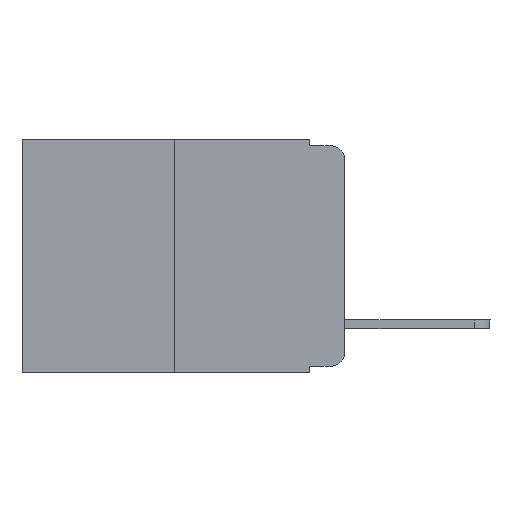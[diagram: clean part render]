
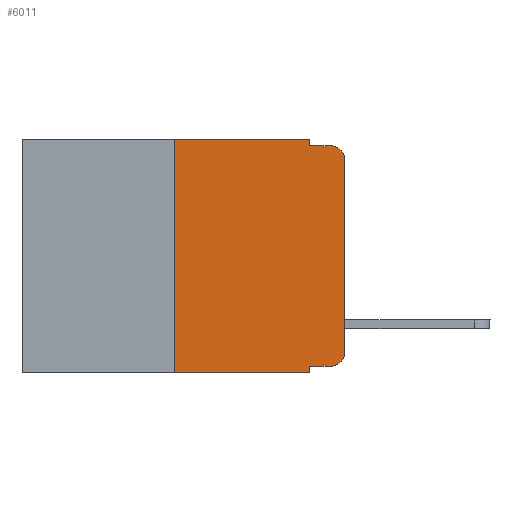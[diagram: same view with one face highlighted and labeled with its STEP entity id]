
A CAD part, left-side view. The second image highlights one B-rep face of the part: STEP entity #6011.
In plain terms, the highlighted planar face has unit normal (-1, 0, 0).
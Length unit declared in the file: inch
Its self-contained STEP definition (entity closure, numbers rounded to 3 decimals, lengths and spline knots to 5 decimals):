
#481 = DIRECTION ( 'NONE',  ( 1., 0., 0. ) ) ;
#560 = EDGE_CURVE ( 'NONE', #4453, #16022, #7278, .T. ) ;
#715 = DIRECTION ( 'NONE',  ( 0., -1., 0. ) ) ;
#880 = DIRECTION ( 'NONE',  ( -1., 0., 0. ) ) ;
#976 = DIRECTION ( 'NONE',  ( -1., 0., 0. ) ) ;
#1226 = LINE ( 'NONE', #1460, #8459 ) ;
#1460 = CARTESIAN_POINT ( 'NONE',  ( 0., 0., 0. ) ) ;
#1486 = CARTESIAN_POINT ( 'NONE',  ( 0., 0.051, -0.01 ) ) ;
#1643 = CARTESIAN_POINT ( 'NONE',  ( 0., 0., -0.313 ) ) ;
#1902 = VERTEX_POINT ( 'NONE', #14314 ) ;
#1941 = VERTEX_POINT ( 'NONE', #1643 ) ;
#2982 = CARTESIAN_POINT ( 'NONE',  ( 0., 0.051, 0. ) ) ;
#3220 = CARTESIAN_POINT ( 'NONE',  ( 0., 0.051, -0.343 ) ) ;
#3945 = ORIENTED_EDGE ( 'NONE', *, *, #18774, .T. ) ;
#4025 = CIRCLE ( 'NONE', #15265, 0.02 ) ;
#4037 = EDGE_CURVE ( 'NONE', #11998, #16022, #5168, .T. ) ;
#4082 = CARTESIAN_POINT ( 'NONE',  ( 0., 0.051, -0.333 ) ) ;
#4453 = VERTEX_POINT ( 'NONE', #7261 ) ;
#4628 = AXIS2_PLACEMENT_3D ( 'NONE', #8307, #976, #11021 ) ;
#4678 = CARTESIAN_POINT ( 'NONE',  ( 0., 0.473, 0. ) ) ;
#4735 = DIRECTION ( 'NONE',  ( 0., -1., 0. ) ) ;
#4806 = VECTOR ( 'NONE', #10927, 39.37008 ) ;
#4898 = ORIENTED_EDGE ( 'NONE', *, *, #4037, .F. ) ;
#5168 = LINE ( 'NONE', #2982, #16307 ) ;
#5452 = VECTOR ( 'NONE', #15469, 39.37008 ) ;
#5868 = DIRECTION ( 'NONE',  ( 0., 0., 1. ) ) ;
#6011 = ADVANCED_FACE ( 'NONE', ( #11650 ), #9129, .F. ) ;
#6039 = ORIENTED_EDGE ( 'NONE', *, *, #10083, .T. ) ;
#6828 = VECTOR ( 'NONE', #4735, 39.37008 ) ;
#7061 = EDGE_CURVE ( 'NONE', #17145, #14745, #8682, .T. ) ;
#7247 = CARTESIAN_POINT ( 'NONE',  ( 0., 0.25, 0. ) ) ;
#7261 = CARTESIAN_POINT ( 'NONE',  ( 0., 0.25, -0.343 ) ) ;
#7278 = LINE ( 'NONE', #18472, #5452 ) ;
#7441 = EDGE_CURVE ( 'NONE', #8144, #17145, #17086, .T. ) ;
#7569 = EDGE_CURVE ( 'NONE', #1941, #1902, #1226, .T. ) ;
#7587 = ORIENTED_EDGE ( 'NONE', *, *, #7441, .F. ) ;
#8144 = VERTEX_POINT ( 'NONE', #7247 ) ;
#8307 = CARTESIAN_POINT ( 'NONE',  ( 0., 0.02, -0.313 ) ) ;
#8459 = VECTOR ( 'NONE', #5868, 39.37008 ) ;
#8682 = LINE ( 'NONE', #12331, #4806 ) ;
#8767 = CARTESIAN_POINT ( 'NONE',  ( 0., 0.02, -0.333 ) ) ;
#8779 = EDGE_CURVE ( 'NONE', #14745, #15457, #15220, .T. ) ;
#9129 = PLANE ( 'NONE',  #13879 ) ;
#9362 = CARTESIAN_POINT ( 'NONE',  ( 0., 0.051, -0.333 ) ) ;
#9684 = CARTESIAN_POINT ( 'NONE',  ( 0., 0.051, 0. ) ) ;
#9891 = LINE ( 'NONE', #9362, #10556 ) ;
#9906 = ORIENTED_EDGE ( 'NONE', *, *, #8779, .F. ) ;
#10083 = EDGE_CURVE ( 'NONE', #1902, #15457, #4025, .T. ) ;
#10556 = VECTOR ( 'NONE', #715, 39.37008 ) ;
#10577 = DIRECTION ( 'NONE',  ( 0., 0., -1. ) ) ;
#10675 = DIRECTION ( 'NONE',  ( 0., -1., 0. ) ) ;
#10725 = ORIENTED_EDGE ( 'NONE', *, *, #13771, .T. ) ;
#10796 = CARTESIAN_POINT ( 'NONE',  ( 0., 0.473, 0. ) ) ;
#10927 = DIRECTION ( 'NONE',  ( 0., 0., -1. ) ) ;
#11021 = DIRECTION ( 'NONE',  ( 0., 0., -1. ) ) ;
#11472 = DIRECTION ( 'NONE',  ( 0., 0., 1. ) ) ;
#11650 = FACE_OUTER_BOUND ( 'NONE', #16495, .T. ) ;
#11998 = VERTEX_POINT ( 'NONE', #4082 ) ;
#12331 = CARTESIAN_POINT ( 'NONE',  ( 0., 0.051, 0. ) ) ;
#12458 = CARTESIAN_POINT ( 'NONE',  ( 0., 0.02, -0.03 ) ) ;
#13091 = LINE ( 'NONE', #14532, #18098 ) ;
#13173 = CARTESIAN_POINT ( 'NONE',  ( 0., 0.051, -0.01 ) ) ;
#13282 = ORIENTED_EDGE ( 'NONE', *, *, #560, .T. ) ;
#13342 = ORIENTED_EDGE ( 'NONE', *, *, #7569, .T. ) ;
#13771 = EDGE_CURVE ( 'NONE', #14607, #1941, #15020, .T. ) ;
#13785 = DIRECTION ( 'NONE',  ( 0., 0., -1. ) ) ;
#13879 = AXIS2_PLACEMENT_3D ( 'NONE', #4678, #481, #10577 ) ;
#14314 = CARTESIAN_POINT ( 'NONE',  ( 0., 0., -0.03 ) ) ;
#14532 = CARTESIAN_POINT ( 'NONE',  ( 0., 0.25, 0. ) ) ;
#14562 = DIRECTION ( 'NONE',  ( 0., 0., -1. ) ) ;
#14607 = VERTEX_POINT ( 'NONE', #8767 ) ;
#14745 = VERTEX_POINT ( 'NONE', #1486 ) ;
#15020 = CIRCLE ( 'NONE', #4628, 0.02 ) ;
#15220 = LINE ( 'NONE', #13173, #6828 ) ;
#15262 = VECTOR ( 'NONE', #10675, 39.37008 ) ;
#15265 = AXIS2_PLACEMENT_3D ( 'NONE', #12458, #880, #13785 ) ;
#15443 = ORIENTED_EDGE ( 'NONE', *, *, #7061, .F. ) ;
#15457 = VERTEX_POINT ( 'NONE', #17568 ) ;
#15469 = DIRECTION ( 'NONE',  ( 0., -1., 0. ) ) ;
#16022 = VERTEX_POINT ( 'NONE', #3220 ) ;
#16307 = VECTOR ( 'NONE', #14562, 39.37008 ) ;
#16495 = EDGE_LOOP ( 'NONE', ( #13342, #6039, #9906, #15443, #7587, #16691, #13282, #4898, #3945, #10725 ) ) ;
#16691 = ORIENTED_EDGE ( 'NONE', *, *, #17949, .F. ) ;
#17086 = LINE ( 'NONE', #10796, #15262 ) ;
#17145 = VERTEX_POINT ( 'NONE', #9684 ) ;
#17568 = CARTESIAN_POINT ( 'NONE',  ( 0., 0.02, -0.01 ) ) ;
#17949 = EDGE_CURVE ( 'NONE', #4453, #8144, #13091, .T. ) ;
#18098 = VECTOR ( 'NONE', #11472, 39.37008 ) ;
#18472 = CARTESIAN_POINT ( 'NONE',  ( 0., 0.473, -0.343 ) ) ;
#18774 = EDGE_CURVE ( 'NONE', #11998, #14607, #9891, .T. ) ;
